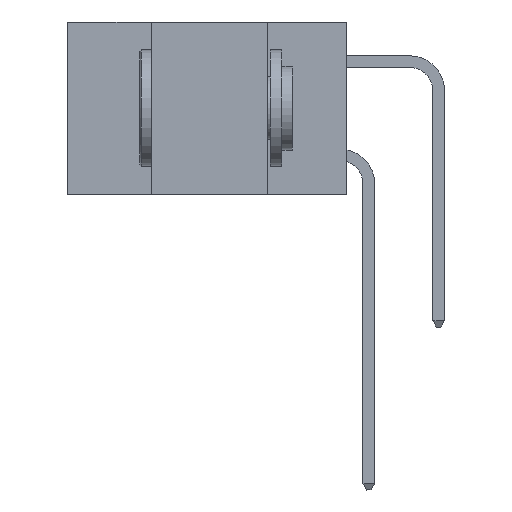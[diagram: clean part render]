
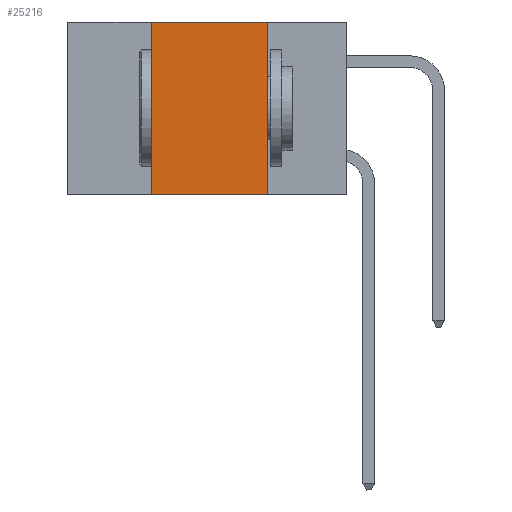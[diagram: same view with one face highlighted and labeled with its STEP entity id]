
A CAD part, left-side view. The second image highlights one B-rep face of the part: STEP entity #25216.
In plain terms, the highlighted planar face has unit normal (-1, 0, 0).
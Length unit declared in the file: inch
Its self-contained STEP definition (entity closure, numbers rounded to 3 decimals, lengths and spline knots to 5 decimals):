
#567 = LINE ( 'NONE', #10649, #20079 ) ;
#1154 = EDGE_CURVE ( 'NONE', #1316, #18216, #567, .T. ) ;
#1316 = VERTEX_POINT ( 'NONE', #32156 ) ;
#1612 = LINE ( 'NONE', #27780, #21124 ) ;
#1693 = CARTESIAN_POINT ( 'NONE',  ( 0., 0.17, 0. ) ) ;
#5304 = ORIENTED_EDGE ( 'NONE', *, *, #16706, .T. ) ;
#5319 = CARTESIAN_POINT ( 'NONE',  ( 0., 0.42, 0. ) ) ;
#6963 = DIRECTION ( 'NONE',  ( 0., -1., 0. ) ) ;
#7656 = CARTESIAN_POINT ( 'NONE',  ( 0., 0.17, 0. ) ) ;
#7770 = VERTEX_POINT ( 'NONE', #24574 ) ;
#7964 = DIRECTION ( 'NONE',  ( 0., 0., 1. ) ) ;
#8883 = AXIS2_PLACEMENT_3D ( 'NONE', #29062, #13885, #31574 ) ;
#9782 = LINE ( 'NONE', #24798, #23361 ) ;
#10319 = DIRECTION ( 'NONE',  ( 0., 0., -1. ) ) ;
#10649 = CARTESIAN_POINT ( 'NONE',  ( 0., 0.42, 0. ) ) ;
#11325 = PLANE ( 'NONE',  #8883 ) ;
#13885 = DIRECTION ( 'NONE',  ( 1., 0., 0. ) ) ;
#14444 = ORIENTED_EDGE ( 'NONE', *, *, #1154, .F. ) ;
#16706 = EDGE_CURVE ( 'NONE', #1316, #7770, #9782, .T. ) ;
#18216 = VERTEX_POINT ( 'NONE', #5319 ) ;
#18700 = EDGE_LOOP ( 'NONE', ( #27111, #32537, #14444, #5304 ) ) ;
#19183 = VECTOR ( 'NONE', #10319, 39.37008 ) ;
#20079 = VECTOR ( 'NONE', #7964, 39.37008 ) ;
#21124 = VECTOR ( 'NONE', #27673, 39.37008 ) ;
#21859 = FACE_OUTER_BOUND ( 'NONE', #18700, .T. ) ;
#22163 = VERTEX_POINT ( 'NONE', #1693 ) ;
#23361 = VECTOR ( 'NONE', #6963, 39.37008 ) ;
#24352 = EDGE_CURVE ( 'NONE', #18216, #22163, #1612, .T. ) ;
#24574 = CARTESIAN_POINT ( 'NONE',  ( 0., 0.17, -0.37 ) ) ;
#24798 = CARTESIAN_POINT ( 'NONE',  ( 0., 0.6, -0.37 ) ) ;
#25216 = ADVANCED_FACE ( 'NONE', ( #21859 ), #11325, .F. ) ;
#26680 = LINE ( 'NONE', #7656, #19183 ) ;
#27111 = ORIENTED_EDGE ( 'NONE', *, *, #31974, .F. ) ;
#27673 = DIRECTION ( 'NONE',  ( 0., -1., 0. ) ) ;
#27780 = CARTESIAN_POINT ( 'NONE',  ( 0., 0.6, 0. ) ) ;
#29062 = CARTESIAN_POINT ( 'NONE',  ( 0., 0.6, 0. ) ) ;
#31574 = DIRECTION ( 'NONE',  ( 0., 0., -1. ) ) ;
#31974 = EDGE_CURVE ( 'NONE', #22163, #7770, #26680, .T. ) ;
#32156 = CARTESIAN_POINT ( 'NONE',  ( 0., 0.42, -0.37 ) ) ;
#32537 = ORIENTED_EDGE ( 'NONE', *, *, #24352, .F. ) ;
